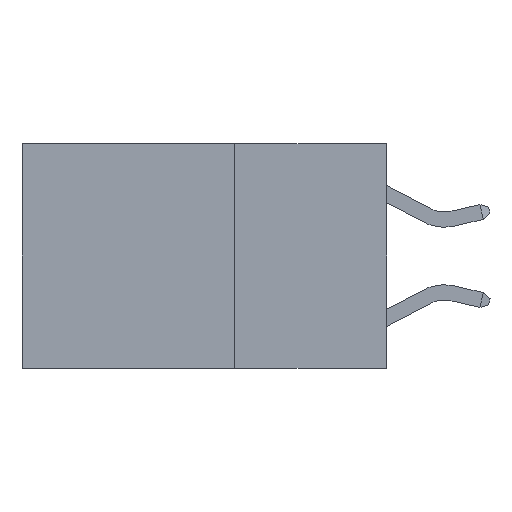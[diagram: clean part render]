
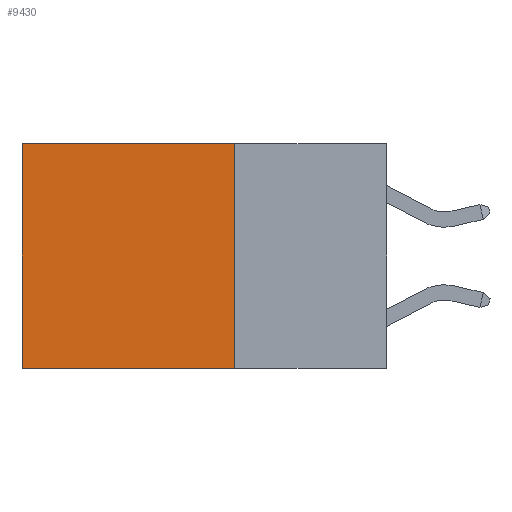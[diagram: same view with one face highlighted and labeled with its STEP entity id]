
A CAD part, left-side view. The second image highlights one B-rep face of the part: STEP entity #9430.
In plain terms, the highlighted planar face has unit normal (-1, 0, 0).
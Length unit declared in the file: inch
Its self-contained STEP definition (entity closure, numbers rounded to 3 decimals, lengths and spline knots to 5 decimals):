
#1406 = CARTESIAN_POINT ( 'NONE',  ( 0.2625, 0.6, 0. ) ) ;
#1599 = DIRECTION ( 'NONE',  ( 0., 0., -1. ) ) ;
#2014 = VECTOR ( 'NONE', #11183, 39.37008 ) ;
#2351 = ORIENTED_EDGE ( 'NONE', *, *, #26983, .T. ) ;
#3129 = CARTESIAN_POINT ( 'NONE',  ( 0.2625, 0.6, -0.37 ) ) ;
#4803 = CARTESIAN_POINT ( 'NONE',  ( 0.2625, 0.25, 0. ) ) ;
#6541 = CARTESIAN_POINT ( 'NONE',  ( 0.2625, 0.6, 0. ) ) ;
#7310 = CARTESIAN_POINT ( 'NONE',  ( 0.2625, 0.25, 0. ) ) ;
#7471 = VERTEX_POINT ( 'NONE', #7310 ) ;
#7931 = DIRECTION ( 'NONE',  ( 0., 1., 0. ) ) ;
#8266 = CARTESIAN_POINT ( 'NONE',  ( 0.2625, 0.25, 0. ) ) ;
#8676 = LINE ( 'NONE', #6541, #14251 ) ;
#9430 = ADVANCED_FACE ( 'NONE', ( #12549 ), #17083, .F. ) ;
#10124 = EDGE_CURVE ( 'NONE', #7471, #12207, #20013, .T. ) ;
#10393 = EDGE_CURVE ( 'NONE', #12207, #11034, #19553, .T. ) ;
#11034 = VERTEX_POINT ( 'NONE', #3129 ) ;
#11183 = DIRECTION ( 'NONE',  ( 0., 1., 0. ) ) ;
#12207 = VERTEX_POINT ( 'NONE', #22840 ) ;
#12385 = ORIENTED_EDGE ( 'NONE', *, *, #10124, .F. ) ;
#12470 = VECTOR ( 'NONE', #22449, 39.37008 ) ;
#12549 = FACE_OUTER_BOUND ( 'NONE', #18903, .T. ) ;
#14251 = VECTOR ( 'NONE', #15227, 39.37008 ) ;
#14347 = LINE ( 'NONE', #27417, #27812 ) ;
#15227 = DIRECTION ( 'NONE',  ( 0., 0., -1. ) ) ;
#16509 = AXIS2_PLACEMENT_3D ( 'NONE', #8266, #25759, #1599 ) ;
#17083 = PLANE ( 'NONE',  #16509 ) ;
#17559 = CARTESIAN_POINT ( 'NONE',  ( 0.2625, 0.25, -0.37 ) ) ;
#18903 = EDGE_LOOP ( 'NONE', ( #2351, #19098, #12385, #21689 ) ) ;
#19098 = ORIENTED_EDGE ( 'NONE', *, *, #10393, .F. ) ;
#19553 = LINE ( 'NONE', #17559, #2014 ) ;
#20013 = LINE ( 'NONE', #4803, #12470 ) ;
#21689 = ORIENTED_EDGE ( 'NONE', *, *, #25462, .T. ) ;
#22449 = DIRECTION ( 'NONE',  ( 0., 0., -1. ) ) ;
#22840 = CARTESIAN_POINT ( 'NONE',  ( 0.2625, 0.25, -0.37 ) ) ;
#25348 = VERTEX_POINT ( 'NONE', #1406 ) ;
#25462 = EDGE_CURVE ( 'NONE', #7471, #25348, #14347, .T. ) ;
#25759 = DIRECTION ( 'NONE',  ( 1., 0., 0. ) ) ;
#26983 = EDGE_CURVE ( 'NONE', #25348, #11034, #8676, .T. ) ;
#27417 = CARTESIAN_POINT ( 'NONE',  ( 0.2625, 0.25, 0. ) ) ;
#27812 = VECTOR ( 'NONE', #7931, 39.37008 ) ;
